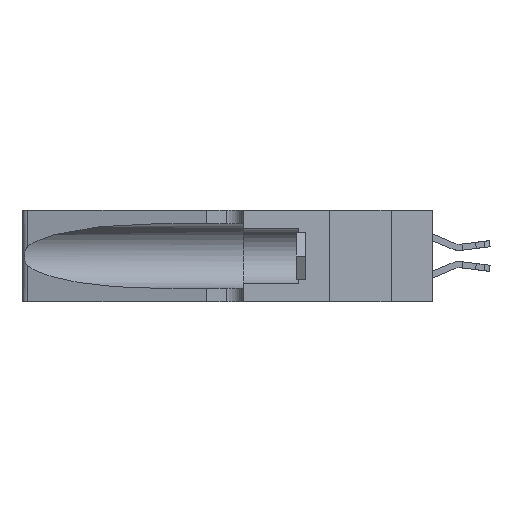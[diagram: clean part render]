
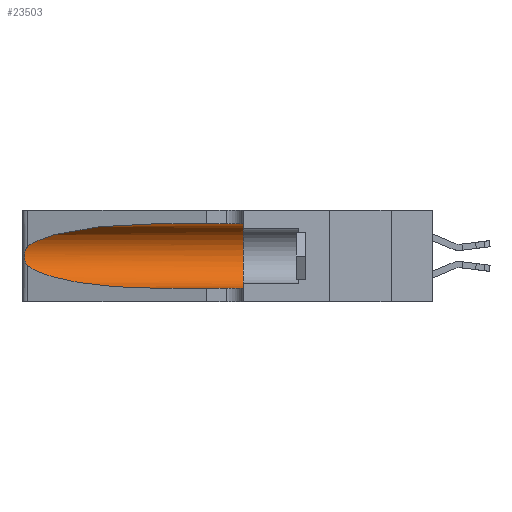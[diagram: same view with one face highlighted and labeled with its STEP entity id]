
A CAD part, left-side view. The second image highlights one B-rep face of the part: STEP entity #23503.
In plain terms, the highlighted cylindrical face has radius 3.308 mm (diameter 6.617 mm), a partial arc.
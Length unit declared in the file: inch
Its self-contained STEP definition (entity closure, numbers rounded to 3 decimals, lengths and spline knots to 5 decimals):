
#244 = DIRECTION ( 'NONE',  ( 0., 1., 0. ) ) ;
#377 = VERTEX_POINT ( 'NONE', #6753 ) ;
#493 = CARTESIAN_POINT ( 'NONE',  ( 0.25854, 1.2359, 0.20912 ) ) ;
#2528 = CARTESIAN_POINT ( 'NONE',  ( 0.26075, 1.23896, 0.19203 ) ) ;
#3731 = CARTESIAN_POINT ( 'NONE',  ( 0.2373, 1.15595, 0.08982 ) ) ;
#4129 = EDGE_LOOP ( 'NONE', ( #18499, #8739, #5734, #15538, #12587, #17570 ) ) ;
#4415 = CARTESIAN_POINT ( 'NONE',  ( 0.25487, 1.22718, 0.22369 ) ) ;
#4586 = CARTESIAN_POINT ( 'NONE',  ( 0.26017, 1.23833, 0.17102 ) ) ;
#4729 = CARTESIAN_POINT ( 'NONE',  ( 0.1305, 0.35, 0.05475 ) ) ;
#5734 = ORIENTED_EDGE ( 'NONE', *, *, #11404, .T. ) ;
#5770 = CARTESIAN_POINT ( 'NONE',  ( 0.25487, 1.22718, 0.14631 ) ) ;
#6322 = B_SPLINE_CURVE_WITH_KNOTS ( 'NONE', 3,
 ( #12495, #22439, #24400, #12576, #493, #14608, #2528, #16598, #4586, #18562, #6610, #20561, #8664, #22515 ),
 .UNSPECIFIED., .F., .F.,
 ( 4, 2, 2, 2, 2, 2, 4 ),
 ( 0., 0.00027, 0.00053, 0.00107, 0.0016, 0.00187, 0.00214 ),
 .UNSPECIFIED. ) ;
#6610 = CARTESIAN_POINT ( 'NONE',  ( 0.25789, 1.23486, 0.15765 ) ) ;
#6753 = CARTESIAN_POINT ( 'NONE',  ( 0.1305, 0.72297, 0.05475 ) ) ;
#7806 = CARTESIAN_POINT ( 'NONE',  ( 0.18966, 0.96281, 0.05475 ) ) ;
#8146 = VECTOR ( 'NONE', #8224, 39.37008 ) ;
#8224 = DIRECTION ( 'NONE',  ( 0., -1., 0. ) ) ;
#8427 = AXIS2_PLACEMENT_3D ( 'NONE', #12343, #244, #14371 ) ;
#8429 = VECTOR ( 'NONE', #22291, 39.37008 ) ;
#8664 = CARTESIAN_POINT ( 'NONE',  ( 0.25555, 1.22993, 0.14849 ) ) ;
#8739 = ORIENTED_EDGE ( 'NONE', *, *, #12220, .T. ) ;
#8937 = CARTESIAN_POINT ( 'NONE',  ( 0.1305, 0.35, 0.31525 ) ) ;
#9174 = CARTESIAN_POINT ( 'NONE',  ( 0.1305, 1.61858, 0.185 ) ) ;
#10428 = CARTESIAN_POINT ( 'NONE',  ( 0.18966, 0.96281, 0.31525 ) ) ;
#10998 =( BOUNDED_CURVE ( )  B_SPLINE_CURVE ( 3, ( #5770, #3731, #7806, #21698 ),
 .UNSPECIFIED., .F., .T. ) 
 B_SPLINE_CURVE_WITH_KNOTS ( ( 4, 4 ),
 ( 3.44316, 4.71239 ),
 .UNSPECIFIED. ) 
 CURVE ( )  GEOMETRIC_REPRESENTATION_ITEM ( )  RATIONAL_B_SPLINE_CURVE ( ( 1., 0.87, 0.87, 1. ) ) 
 REPRESENTATION_ITEM ( '' )  );
#11036 = VERTEX_POINT ( 'NONE', #12630 ) ;
#11256 = AXIS2_PLACEMENT_3D ( 'NONE', #9174, #13164, #21055 ) ;
#11404 = EDGE_CURVE ( 'NONE', #11036, #377, #10998, .T. ) ;
#11591 = CYLINDRICAL_SURFACE ( 'NONE', #11256, 0.13025 ) ;
#12220 = EDGE_CURVE ( 'NONE', #24497, #11036, #6322, .T. ) ;
#12343 = CARTESIAN_POINT ( 'NONE',  ( 0.1305, 0.35, 0.185 ) ) ;
#12423 = CARTESIAN_POINT ( 'NONE',  ( 0.1305, 1.61858, 0.05475 ) ) ;
#12458 = CIRCLE ( 'NONE', #8427, 0.13025 ) ;
#12495 = CARTESIAN_POINT ( 'NONE',  ( 0.25487, 1.22718, 0.22369 ) ) ;
#12576 = CARTESIAN_POINT ( 'NONE',  ( 0.25787, 1.23484, 0.2124 ) ) ;
#12587 = ORIENTED_EDGE ( 'NONE', *, *, #24560, .F. ) ;
#12630 = CARTESIAN_POINT ( 'NONE',  ( 0.25487, 1.22718, 0.14631 ) ) ;
#13164 = DIRECTION ( 'NONE',  ( 0., -1., 0. ) ) ;
#13650 = VERTEX_POINT ( 'NONE', #23847 ) ;
#14277 = CARTESIAN_POINT ( 'NONE',  ( 0.1305, 1.61858, 0.31525 ) ) ;
#14371 = DIRECTION ( 'NONE',  ( 0., 0., 1. ) ) ;
#14608 = CARTESIAN_POINT ( 'NONE',  ( 0.26018, 1.23835, 0.19895 ) ) ;
#15538 = ORIENTED_EDGE ( 'NONE', *, *, #16908, .T. ) ;
#16299 = EDGE_CURVE ( 'NONE', #13650, #25605, #25803, .T. ) ;
#16350 = EDGE_CURVE ( 'NONE', #13650, #24497, #18309, .T. ) ;
#16447 = CARTESIAN_POINT ( 'NONE',  ( 0.2373, 1.15595, 0.28018 ) ) ;
#16598 = CARTESIAN_POINT ( 'NONE',  ( 0.26075, 1.23896, 0.178 ) ) ;
#16908 = EDGE_CURVE ( 'NONE', #377, #20167, #19001, .T. ) ;
#17570 = ORIENTED_EDGE ( 'NONE', *, *, #16299, .F. ) ;
#18065 = CARTESIAN_POINT ( 'NONE',  ( 0.25487, 1.22718, 0.22369 ) ) ;
#18309 =( BOUNDED_CURVE ( )  B_SPLINE_CURVE ( 3, ( #18319, #10428, #16447, #4415 ),
 .UNSPECIFIED., .F., .F. ) 
 B_SPLINE_CURVE_WITH_KNOTS ( ( 4, 4 ),
 ( 1.5708, 2.84003 ),
 .UNSPECIFIED. ) 
 CURVE ( )  GEOMETRIC_REPRESENTATION_ITEM ( )  RATIONAL_B_SPLINE_CURVE ( ( 1., 0.87, 0.87, 1. ) ) 
 REPRESENTATION_ITEM ( '' )  );
#18319 = CARTESIAN_POINT ( 'NONE',  ( 0.1305, 0.72297, 0.31525 ) ) ;
#18499 = ORIENTED_EDGE ( 'NONE', *, *, #16350, .T. ) ;
#18562 = CARTESIAN_POINT ( 'NONE',  ( 0.25856, 1.23593, 0.16098 ) ) ;
#19001 = LINE ( 'NONE', #12423, #8429 ) ;
#20167 = VERTEX_POINT ( 'NONE', #4729 ) ;
#20561 = CARTESIAN_POINT ( 'NONE',  ( 0.25639, 1.23186, 0.15144 ) ) ;
#21055 = DIRECTION ( 'NONE',  ( 0., 0., -1. ) ) ;
#21698 = CARTESIAN_POINT ( 'NONE',  ( 0.1305, 0.72297, 0.05475 ) ) ;
#22118 = FACE_OUTER_BOUND ( 'NONE', #4129, .T. ) ;
#22291 = DIRECTION ( 'NONE',  ( 0., -1., 0. ) ) ;
#22439 = CARTESIAN_POINT ( 'NONE',  ( 0.25555, 1.22994, 0.2215 ) ) ;
#22515 = CARTESIAN_POINT ( 'NONE',  ( 0.25487, 1.22718, 0.14631 ) ) ;
#23503 = ADVANCED_FACE ( 'NONE', ( #22118 ), #11591, .F. ) ;
#23847 = CARTESIAN_POINT ( 'NONE',  ( 0.1305, 0.72297, 0.31525 ) ) ;
#24400 = CARTESIAN_POINT ( 'NONE',  ( 0.25639, 1.23184, 0.21858 ) ) ;
#24497 = VERTEX_POINT ( 'NONE', #18065 ) ;
#24560 = EDGE_CURVE ( 'NONE', #25605, #20167, #12458, .T. ) ;
#25605 = VERTEX_POINT ( 'NONE', #8937 ) ;
#25803 = LINE ( 'NONE', #14277, #8146 ) ;
